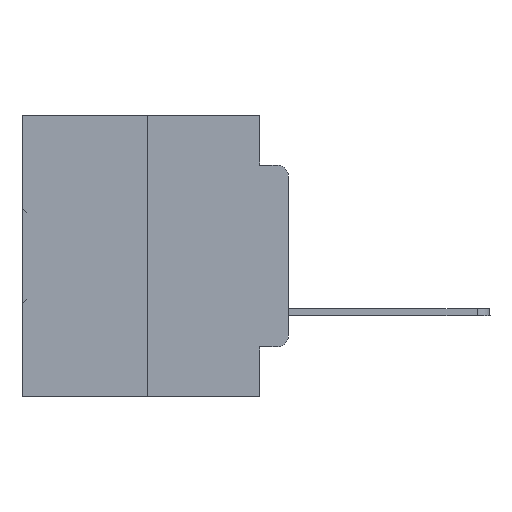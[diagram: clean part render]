
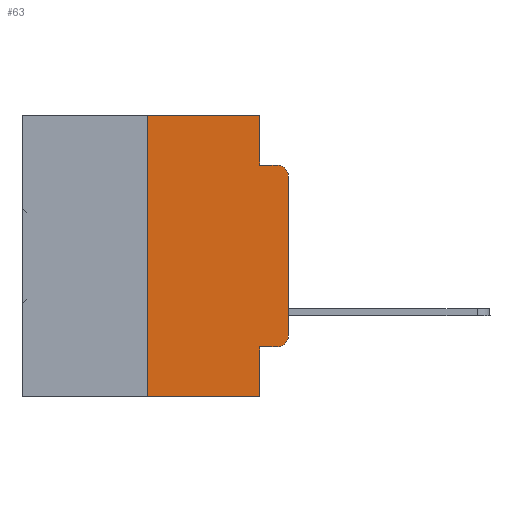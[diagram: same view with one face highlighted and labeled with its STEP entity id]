
A CAD part, left-side view. The second image highlights one B-rep face of the part: STEP entity #63.
In plain terms, the highlighted planar face has unit normal (-1, 0, 0).
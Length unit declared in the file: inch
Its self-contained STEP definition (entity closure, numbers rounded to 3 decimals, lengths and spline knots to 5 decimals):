
#63 = ADVANCED_FACE ( 'NONE', ( #3347 ), #27770, .F. ) ;
#1238 = CARTESIAN_POINT ( 'NONE',  ( 0., 0.051, 0. ) ) ;
#1292 = VERTEX_POINT ( 'NONE', #28209 ) ;
#1387 = VECTOR ( 'NONE', #6577, 39.37008 ) ;
#1945 = VERTEX_POINT ( 'NONE', #5709 ) ;
#1997 = VECTOR ( 'NONE', #25217, 39.37008 ) ;
#2046 = AXIS2_PLACEMENT_3D ( 'NONE', #22852, #14924, #28370 ) ;
#2280 = CARTESIAN_POINT ( 'NONE',  ( 0., 0.051, 0. ) ) ;
#3347 = FACE_OUTER_BOUND ( 'NONE', #23571, .T. ) ;
#3826 = VERTEX_POINT ( 'NONE', #9069 ) ;
#4299 = CARTESIAN_POINT ( 'NONE',  ( 0., 0.051, 0. ) ) ;
#4840 = ORIENTED_EDGE ( 'NONE', *, *, #17632, .T. ) ;
#5133 = EDGE_CURVE ( 'NONE', #24781, #9994, #20446, .T. ) ;
#5447 = VECTOR ( 'NONE', #18875, 39.37008 ) ;
#5471 = CARTESIAN_POINT ( 'NONE',  ( 0., 0.051, -0.4115 ) ) ;
#5709 = CARTESIAN_POINT ( 'NONE',  ( 0., 0., -0.3915 ) ) ;
#5969 = DIRECTION ( 'NONE',  ( 0., 0., -1. ) ) ;
#6327 = DIRECTION ( 'NONE',  ( -1., 0., 0. ) ) ;
#6563 = ORIENTED_EDGE ( 'NONE', *, *, #20230, .T. ) ;
#6577 = DIRECTION ( 'NONE',  ( 0., 0., 1. ) ) ;
#6677 = LINE ( 'NONE', #33465, #1997 ) ;
#6762 = EDGE_CURVE ( 'NONE', #11308, #21224, #31987, .T. ) ;
#6779 = CARTESIAN_POINT ( 'NONE',  ( 0., 0.02, -0.0885 ) ) ;
#7483 = AXIS2_PLACEMENT_3D ( 'NONE', #11284, #11176, #30369 ) ;
#7504 = ORIENTED_EDGE ( 'NONE', *, *, #8974, .F. ) ;
#7799 = VECTOR ( 'NONE', #34435, 39.37008 ) ;
#8247 = DIRECTION ( 'NONE',  ( 0., -1., 0. ) ) ;
#8882 = LINE ( 'NONE', #17631, #14141 ) ;
#8912 = CIRCLE ( 'NONE', #10979, 0.02 ) ;
#8974 = EDGE_CURVE ( 'NONE', #1292, #34017, #14155, .T. ) ;
#9069 = CARTESIAN_POINT ( 'NONE',  ( 0., 0.02, -0.4115 ) ) ;
#9213 = VERTEX_POINT ( 'NONE', #12161 ) ;
#9994 = VERTEX_POINT ( 'NONE', #6779 ) ;
#10791 = CARTESIAN_POINT ( 'NONE',  ( 0., 0.051, -0.0885 ) ) ;
#10905 = EDGE_CURVE ( 'NONE', #32381, #1292, #8882, .T. ) ;
#10979 = AXIS2_PLACEMENT_3D ( 'NONE', #22698, #6327, #5969 ) ;
#11134 = ORIENTED_EDGE ( 'NONE', *, *, #29015, .T. ) ;
#11176 = DIRECTION ( 'NONE',  ( 1., 0., 0. ) ) ;
#11284 = CARTESIAN_POINT ( 'NONE',  ( 0., 0.473, 0. ) ) ;
#11308 = VERTEX_POINT ( 'NONE', #5471 ) ;
#12161 = CARTESIAN_POINT ( 'NONE',  ( 0., 0., -0.1085 ) ) ;
#12438 = VECTOR ( 'NONE', #35597, 39.37008 ) ;
#14141 = VECTOR ( 'NONE', #23280, 39.37008 ) ;
#14155 = LINE ( 'NONE', #25331, #20192 ) ;
#14924 = DIRECTION ( 'NONE',  ( -1., 0., 0. ) ) ;
#16441 = LINE ( 'NONE', #20313, #1387 ) ;
#16579 = EDGE_CURVE ( 'NONE', #3826, #1945, #18908, .T. ) ;
#17186 = DIRECTION ( 'NONE',  ( 0., -1., 0. ) ) ;
#17631 = CARTESIAN_POINT ( 'NONE',  ( 0., 0.25, 0. ) ) ;
#17632 = EDGE_CURVE ( 'NONE', #9213, #9994, #8912, .T. ) ;
#18605 = CARTESIAN_POINT ( 'NONE',  ( 0., 0.25, -0.5 ) ) ;
#18875 = DIRECTION ( 'NONE',  ( 0., 0., -1. ) ) ;
#18908 = CIRCLE ( 'NONE', #2046, 0.02 ) ;
#19125 = ORIENTED_EDGE ( 'NONE', *, *, #10905, .F. ) ;
#19175 = VECTOR ( 'NONE', #8247, 39.37008 ) ;
#20192 = VECTOR ( 'NONE', #17186, 39.37008 ) ;
#20230 = EDGE_CURVE ( 'NONE', #11308, #3826, #6677, .T. ) ;
#20313 = CARTESIAN_POINT ( 'NONE',  ( 0., 0., 0. ) ) ;
#20446 = LINE ( 'NONE', #10791, #19175 ) ;
#20698 = ORIENTED_EDGE ( 'NONE', *, *, #16579, .T. ) ;
#21080 = ORIENTED_EDGE ( 'NONE', *, *, #24502, .F. ) ;
#21111 = ORIENTED_EDGE ( 'NONE', *, *, #6762, .F. ) ;
#21224 = VERTEX_POINT ( 'NONE', #32919 ) ;
#22698 = CARTESIAN_POINT ( 'NONE',  ( 0., 0.02, -0.1085 ) ) ;
#22852 = CARTESIAN_POINT ( 'NONE',  ( 0., 0.02, -0.3915 ) ) ;
#23280 = DIRECTION ( 'NONE',  ( 0., 0., 1. ) ) ;
#23571 = EDGE_LOOP ( 'NONE', ( #27573, #4840, #32535, #21080, #7504, #19125, #11134, #21111, #6563, #20698 ) ) ;
#24502 = EDGE_CURVE ( 'NONE', #34017, #24781, #33909, .T. ) ;
#24781 = VERTEX_POINT ( 'NONE', #26902 ) ;
#25217 = DIRECTION ( 'NONE',  ( 0., -1., 0. ) ) ;
#25331 = CARTESIAN_POINT ( 'NONE',  ( 0., 0.473, 0. ) ) ;
#26902 = CARTESIAN_POINT ( 'NONE',  ( 0., 0.051, -0.0885 ) ) ;
#27573 = ORIENTED_EDGE ( 'NONE', *, *, #31708, .T. ) ;
#27770 = PLANE ( 'NONE',  #7483 ) ;
#28209 = CARTESIAN_POINT ( 'NONE',  ( 0., 0.25, 0. ) ) ;
#28370 = DIRECTION ( 'NONE',  ( 0., 0., -1. ) ) ;
#29015 = EDGE_CURVE ( 'NONE', #32381, #21224, #34858, .T. ) ;
#30369 = DIRECTION ( 'NONE',  ( 0., 0., -1. ) ) ;
#31708 = EDGE_CURVE ( 'NONE', #1945, #9213, #16441, .T. ) ;
#31987 = LINE ( 'NONE', #4299, #7799 ) ;
#32381 = VERTEX_POINT ( 'NONE', #18605 ) ;
#32535 = ORIENTED_EDGE ( 'NONE', *, *, #5133, .F. ) ;
#32919 = CARTESIAN_POINT ( 'NONE',  ( 0., 0.051, -0.5 ) ) ;
#32951 = CARTESIAN_POINT ( 'NONE',  ( 0., 0.473, -0.5 ) ) ;
#33465 = CARTESIAN_POINT ( 'NONE',  ( 0., 0.051, -0.4115 ) ) ;
#33909 = LINE ( 'NONE', #2280, #5447 ) ;
#34017 = VERTEX_POINT ( 'NONE', #1238 ) ;
#34435 = DIRECTION ( 'NONE',  ( 0., 0., -1. ) ) ;
#34858 = LINE ( 'NONE', #32951, #12438 ) ;
#35597 = DIRECTION ( 'NONE',  ( 0., -1., 0. ) ) ;
